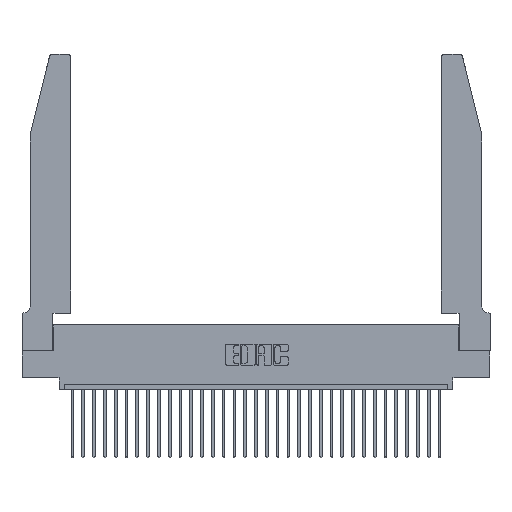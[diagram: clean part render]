
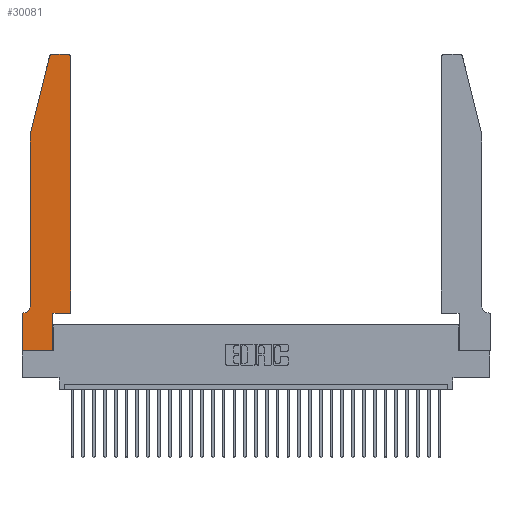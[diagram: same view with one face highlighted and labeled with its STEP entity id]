
A CAD part, top view. The second image highlights one B-rep face of the part: STEP entity #30081.
In plain terms, the highlighted planar face has unit normal (0, 0, 1).
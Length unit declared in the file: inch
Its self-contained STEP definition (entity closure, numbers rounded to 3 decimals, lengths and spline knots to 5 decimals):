
#347 = DIRECTION ( 'NONE',  ( 0., -1., 0. ) ) ;
#744 = LINE ( 'NONE', #11428, #8475 ) ;
#945 = VERTEX_POINT ( 'NONE', #5256 ) ;
#1179 = FACE_OUTER_BOUND ( 'NONE', #5903, .T. ) ;
#1496 = DIRECTION ( 'NONE',  ( 0., 0., 1. ) ) ;
#1560 = ORIENTED_EDGE ( 'NONE', *, *, #28983, .T. ) ;
#1597 = DIRECTION ( 'NONE',  ( 1., 0., 0. ) ) ;
#2192 = ORIENTED_EDGE ( 'NONE', *, *, #10754, .T. ) ;
#2549 = LINE ( 'NONE', #15662, #13070 ) ;
#2661 = CIRCLE ( 'NONE', #5940, 0.07 ) ;
#3040 = LINE ( 'NONE', #4334, #27112 ) ;
#3099 = VERTEX_POINT ( 'NONE', #30598 ) ;
#3325 = DIRECTION ( 'NONE',  ( 1., 0., 0. ) ) ;
#3476 = VERTEX_POINT ( 'NONE', #14508 ) ;
#3698 = EDGE_CURVE ( 'NONE', #27173, #24502, #744, .T. ) ;
#3827 = DIRECTION ( 'NONE',  ( 1., 0., 0. ) ) ;
#4166 = DIRECTION ( 'NONE',  ( 0., 1., 0. ) ) ;
#4210 = DIRECTION ( 'NONE',  ( -0.239, -0.971, 0. ) ) ;
#4315 = VERTEX_POINT ( 'NONE', #25001 ) ;
#4334 = CARTESIAN_POINT ( 'NONE',  ( 0., 0., 0.37 ) ) ;
#4410 = LINE ( 'NONE', #8948, #31168 ) ;
#4447 = DIRECTION ( 'NONE',  ( 0., -1., 0. ) ) ;
#4910 = AXIS2_PLACEMENT_3D ( 'NONE', #23759, #1496, #1597 ) ;
#4913 = EDGE_CURVE ( 'NONE', #18213, #3099, #22873, .T. ) ;
#5014 = VECTOR ( 'NONE', #20845, 39.37008 ) ;
#5217 = CARTESIAN_POINT ( 'NONE',  ( 0.4205, 2.72, 0.37 ) ) ;
#5256 = CARTESIAN_POINT ( 'NONE',  ( 0.0055, 0.35, 0.37 ) ) ;
#5903 = EDGE_LOOP ( 'NONE', ( #26340, #17524, #26783, #25759, #2192, #11421, #29727, #32034, #14233, #11478, #1560, #26995 ) ) ;
#5940 = AXIS2_PLACEMENT_3D ( 'NONE', #26116, #11260, #28634 ) ;
#6091 = LINE ( 'NONE', #32172, #31370 ) ;
#6135 = EDGE_CURVE ( 'NONE', #4315, #27924, #2549, .T. ) ;
#7097 = AXIS2_PLACEMENT_3D ( 'NONE', #5217, #15220, #17721 ) ;
#7296 = CARTESIAN_POINT ( 'NONE',  ( 0.0755, 0.42, 0.37 ) ) ;
#8475 = VECTOR ( 'NONE', #3827, 39.37008 ) ;
#8948 = CARTESIAN_POINT ( 'NONE',  ( 0.4505, 0.35, 0.37 ) ) ;
#10069 = EDGE_CURVE ( 'NONE', #19376, #15621, #21017, .T. ) ;
#10754 = EDGE_CURVE ( 'NONE', #27924, #945, #2661, .T. ) ;
#11116 = EDGE_CURVE ( 'NONE', #29630, #27173, #3040, .T. ) ;
#11260 = DIRECTION ( 'NONE',  ( 0., 0., -1. ) ) ;
#11421 = ORIENTED_EDGE ( 'NONE', *, *, #25647, .T. ) ;
#11428 = CARTESIAN_POINT ( 'NONE',  ( 0., 0., 0.37 ) ) ;
#11478 = ORIENTED_EDGE ( 'NONE', *, *, #12243, .T. ) ;
#11808 = EDGE_CURVE ( 'NONE', #24502, #3476, #6091, .T. ) ;
#12243 = EDGE_CURVE ( 'NONE', #3476, #14121, #23940, .T. ) ;
#12253 = CARTESIAN_POINT ( 'NONE',  ( 0.2605, 2.75, 0.37 ) ) ;
#12941 = CARTESIAN_POINT ( 'NONE',  ( 0.4505, 0.35, 0.37 ) ) ;
#13070 = VECTOR ( 'NONE', #347, 39.37008 ) ;
#13104 = VECTOR ( 'NONE', #18052, 39.37008 ) ;
#13515 = VECTOR ( 'NONE', #4210, 39.37008 ) ;
#14121 = VERTEX_POINT ( 'NONE', #21489 ) ;
#14220 = CARTESIAN_POINT ( 'NONE',  ( 0.0755, 2., 0.37 ) ) ;
#14233 = ORIENTED_EDGE ( 'NONE', *, *, #11808, .T. ) ;
#14281 = LINE ( 'NONE', #14220, #13515 ) ;
#14508 = CARTESIAN_POINT ( 'NONE',  ( 0.2865, 0.35, 0.37 ) ) ;
#14934 = CARTESIAN_POINT ( 'NONE',  ( 0.4505, 2.72, 0.37 ) ) ;
#15220 = DIRECTION ( 'NONE',  ( 0., 0., 1. ) ) ;
#15621 = VERTEX_POINT ( 'NONE', #21761 ) ;
#15662 = CARTESIAN_POINT ( 'NONE',  ( 0.0755, 2., 0.37 ) ) ;
#17524 = ORIENTED_EDGE ( 'NONE', *, *, #10069, .T. ) ;
#17721 = DIRECTION ( 'NONE',  ( 1., 0., 0. ) ) ;
#18052 = DIRECTION ( 'NONE',  ( 1., 0., 0. ) ) ;
#18213 = VERTEX_POINT ( 'NONE', #14934 ) ;
#18437 = DIRECTION ( 'NONE',  ( 0., 0., 1. ) ) ;
#18536 = CARTESIAN_POINT ( 'NONE',  ( 0.0755, 0.35, 0.37 ) ) ;
#19070 = EDGE_CURVE ( 'NONE', #3099, #19376, #20221, .T. ) ;
#19376 = VERTEX_POINT ( 'NONE', #25674 ) ;
#20221 = LINE ( 'NONE', #12253, #31857 ) ;
#20522 = PLANE ( 'NONE',  #22379 ) ;
#20845 = DIRECTION ( 'NONE',  ( -1., 0., 0. ) ) ;
#20944 = CARTESIAN_POINT ( 'NONE',  ( 0., 0.35, 0.37 ) ) ;
#21017 = CIRCLE ( 'NONE', #4910, 0.03 ) ;
#21489 = CARTESIAN_POINT ( 'NONE',  ( 0.4505, 0.35, 0.37 ) ) ;
#21761 = CARTESIAN_POINT ( 'NONE',  ( 0.25487, 2.72718, 0.37 ) ) ;
#22152 = LINE ( 'NONE', #18536, #5014 ) ;
#22379 = AXIS2_PLACEMENT_3D ( 'NONE', #20944, #18437, #3325 ) ;
#22873 = CIRCLE ( 'NONE', #7097, 0.03 ) ;
#23196 = DIRECTION ( 'NONE',  ( 0., 1., 0. ) ) ;
#23344 = CARTESIAN_POINT ( 'NONE',  ( 0., 0.35, 0.37 ) ) ;
#23610 = CARTESIAN_POINT ( 'NONE',  ( 0., 0., 0.37 ) ) ;
#23759 = CARTESIAN_POINT ( 'NONE',  ( 0.284, 2.72, 0.37 ) ) ;
#23940 = LINE ( 'NONE', #12941, #13104 ) ;
#24502 = VERTEX_POINT ( 'NONE', #26959 ) ;
#25001 = CARTESIAN_POINT ( 'NONE',  ( 0.0755, 2., 0.37 ) ) ;
#25647 = EDGE_CURVE ( 'NONE', #945, #29630, #22152, .T. ) ;
#25674 = CARTESIAN_POINT ( 'NONE',  ( 0.284, 2.75, 0.37 ) ) ;
#25759 = ORIENTED_EDGE ( 'NONE', *, *, #6135, .T. ) ;
#26116 = CARTESIAN_POINT ( 'NONE',  ( 0.0055, 0.42, 0.37 ) ) ;
#26340 = ORIENTED_EDGE ( 'NONE', *, *, #19070, .T. ) ;
#26783 = ORIENTED_EDGE ( 'NONE', *, *, #31467, .T. ) ;
#26959 = CARTESIAN_POINT ( 'NONE',  ( 0.2865, 0., 0.37 ) ) ;
#26995 = ORIENTED_EDGE ( 'NONE', *, *, #4913, .T. ) ;
#27112 = VECTOR ( 'NONE', #4447, 39.37008 ) ;
#27173 = VERTEX_POINT ( 'NONE', #23610 ) ;
#27924 = VERTEX_POINT ( 'NONE', #7296 ) ;
#28634 = DIRECTION ( 'NONE',  ( -1., 0., 0. ) ) ;
#28983 = EDGE_CURVE ( 'NONE', #14121, #18213, #4410, .T. ) ;
#29622 = DIRECTION ( 'NONE',  ( -1., 0., 0. ) ) ;
#29630 = VERTEX_POINT ( 'NONE', #23344 ) ;
#29727 = ORIENTED_EDGE ( 'NONE', *, *, #11116, .T. ) ;
#30081 = ADVANCED_FACE ( 'NONE', ( #1179 ), #20522, .T. ) ;
#30598 = CARTESIAN_POINT ( 'NONE',  ( 0.4205, 2.75, 0.37 ) ) ;
#31168 = VECTOR ( 'NONE', #4166, 39.37008 ) ;
#31370 = VECTOR ( 'NONE', #23196, 39.37008 ) ;
#31467 = EDGE_CURVE ( 'NONE', #15621, #4315, #14281, .T. ) ;
#31857 = VECTOR ( 'NONE', #29622, 39.37008 ) ;
#32034 = ORIENTED_EDGE ( 'NONE', *, *, #3698, .T. ) ;
#32172 = CARTESIAN_POINT ( 'NONE',  ( 0.2865, 0.35, 0.37 ) ) ;
